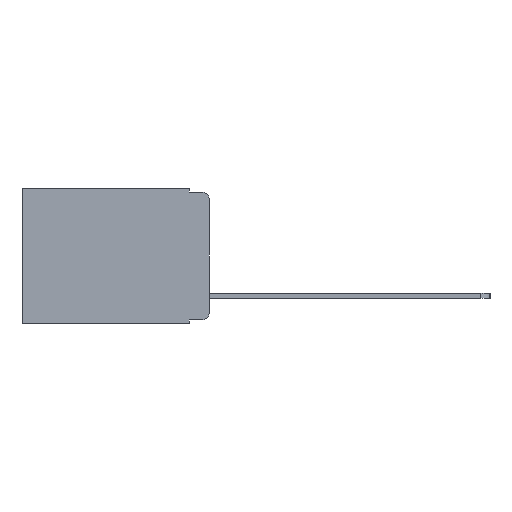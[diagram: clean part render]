
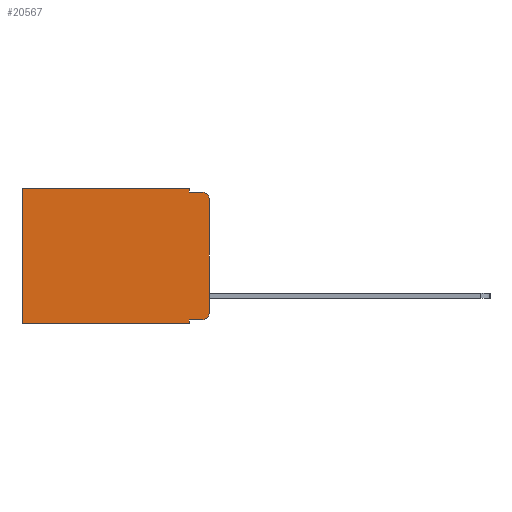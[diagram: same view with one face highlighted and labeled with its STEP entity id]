
A CAD part, left-side view. The second image highlights one B-rep face of the part: STEP entity #20567.
In plain terms, the highlighted planar face has unit normal (-1, 0, 0).
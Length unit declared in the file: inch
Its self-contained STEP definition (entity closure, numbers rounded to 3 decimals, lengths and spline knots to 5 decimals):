
#244 = PLANE ( 'NONE',  #8494 ) ;
#344 = CARTESIAN_POINT ( 'NONE',  ( 0.298, 0.473, 0. ) ) ;
#379 = CARTESIAN_POINT ( 'NONE',  ( 0.298, 0.051, -0.333 ) ) ;
#844 = EDGE_CURVE ( 'NONE', #4341, #19046, #16260, .T. ) ;
#887 = VECTOR ( 'NONE', #14789, 39.37008 ) ;
#1868 = VECTOR ( 'NONE', #18567, 39.37008 ) ;
#2318 = LINE ( 'NONE', #379, #11775 ) ;
#2356 = VERTEX_POINT ( 'NONE', #9933 ) ;
#2668 = DIRECTION ( 'NONE',  ( -1., 0., 0. ) ) ;
#3443 = VECTOR ( 'NONE', #21147, 39.37008 ) ;
#3569 = EDGE_LOOP ( 'NONE', ( #6700, #14458, #13528, #19645, #6907, #20405, #20535, #8109, #5066, #17467 ) ) ;
#4010 = EDGE_CURVE ( 'NONE', #9121, #9765, #20367, .T. ) ;
#4024 = LINE ( 'NONE', #5365, #3443 ) ;
#4341 = VERTEX_POINT ( 'NONE', #8606 ) ;
#4389 = FACE_OUTER_BOUND ( 'NONE', #3569, .T. ) ;
#4958 = CARTESIAN_POINT ( 'NONE',  ( 0.298, 0., 0. ) ) ;
#5066 = ORIENTED_EDGE ( 'NONE', *, *, #10896, .T. ) ;
#5077 = LINE ( 'NONE', #14266, #9252 ) ;
#5365 = CARTESIAN_POINT ( 'NONE',  ( 0.298, 0.473, 0. ) ) ;
#5915 = CARTESIAN_POINT ( 'NONE',  ( 0.298, 0., 0. ) ) ;
#6118 = CARTESIAN_POINT ( 'NONE',  ( 0.298, 0.051, -0.343 ) ) ;
#6130 = VERTEX_POINT ( 'NONE', #8306 ) ;
#6518 = VECTOR ( 'NONE', #14346, 39.37008 ) ;
#6700 = ORIENTED_EDGE ( 'NONE', *, *, #844, .F. ) ;
#6907 = ORIENTED_EDGE ( 'NONE', *, *, #4010, .T. ) ;
#7292 = CARTESIAN_POINT ( 'NONE',  ( 0.298, 0.02, -0.01 ) ) ;
#7557 = CARTESIAN_POINT ( 'NONE',  ( 0.298, 0., 0. ) ) ;
#7899 = DIRECTION ( 'NONE',  ( -1., 0., 0. ) ) ;
#8109 = ORIENTED_EDGE ( 'NONE', *, *, #12081, .F. ) ;
#8306 = CARTESIAN_POINT ( 'NONE',  ( 0.298, 0.051, -0.333 ) ) ;
#8329 = VERTEX_POINT ( 'NONE', #10841 ) ;
#8494 = AXIS2_PLACEMENT_3D ( 'NONE', #7557, #19866, #9335 ) ;
#8558 = EDGE_CURVE ( 'NONE', #8329, #19046, #20690, .T. ) ;
#8606 = CARTESIAN_POINT ( 'NONE',  ( 0.298, 0., -0.03 ) ) ;
#9121 = VERTEX_POINT ( 'NONE', #21879 ) ;
#9252 = VECTOR ( 'NONE', #12483, 39.37008 ) ;
#9256 = VERTEX_POINT ( 'NONE', #6118 ) ;
#9335 = DIRECTION ( 'NONE',  ( 0., 0., -1. ) ) ;
#9765 = VERTEX_POINT ( 'NONE', #344 ) ;
#9933 = CARTESIAN_POINT ( 'NONE',  ( 0.298, 0.473, -0.343 ) ) ;
#10841 = CARTESIAN_POINT ( 'NONE',  ( 0.298, 0.02, -0.333 ) ) ;
#10896 = EDGE_CURVE ( 'NONE', #6130, #8329, #2318, .T. ) ;
#11553 = VECTOR ( 'NONE', #13019, 39.37008 ) ;
#11775 = VECTOR ( 'NONE', #12902, 39.37008 ) ;
#12081 = EDGE_CURVE ( 'NONE', #6130, #9256, #5077, .T. ) ;
#12270 = CARTESIAN_POINT ( 'NONE',  ( 0.298, 0., -0.313 ) ) ;
#12402 = VERTEX_POINT ( 'NONE', #20801 ) ;
#12483 = DIRECTION ( 'NONE',  ( 0., 0., -1. ) ) ;
#12562 = CARTESIAN_POINT ( 'NONE',  ( 0.298, 0.051, 0. ) ) ;
#12902 = DIRECTION ( 'NONE',  ( 0., -1., 0. ) ) ;
#13019 = DIRECTION ( 'NONE',  ( 0., 0., -1. ) ) ;
#13246 = CARTESIAN_POINT ( 'NONE',  ( 0.298, 0.051, -0.01 ) ) ;
#13308 = CARTESIAN_POINT ( 'NONE',  ( 0.298, 0.02, -0.313 ) ) ;
#13528 = ORIENTED_EDGE ( 'NONE', *, *, #19177, .F. ) ;
#14266 = CARTESIAN_POINT ( 'NONE',  ( 0.298, 0.051, 0. ) ) ;
#14346 = DIRECTION ( 'NONE',  ( 0., 0., -1. ) ) ;
#14458 = ORIENTED_EDGE ( 'NONE', *, *, #20362, .T. ) ;
#14789 = DIRECTION ( 'NONE',  ( 0., 1., 0. ) ) ;
#15082 = DIRECTION ( 'NONE',  ( 0., 0., -1. ) ) ;
#15508 = LINE ( 'NONE', #13246, #1868 ) ;
#15643 = EDGE_CURVE ( 'NONE', #9765, #2356, #4024, .T. ) ;
#15865 = CARTESIAN_POINT ( 'NONE',  ( 0.298, 0., -0.343 ) ) ;
#15909 = LINE ( 'NONE', #12562, #6518 ) ;
#15942 = DIRECTION ( 'NONE',  ( 0., 1., 0. ) ) ;
#16016 = AXIS2_PLACEMENT_3D ( 'NONE', #18449, #7899, #20206 ) ;
#16260 = LINE ( 'NONE', #4958, #11553 ) ;
#16822 = EDGE_CURVE ( 'NONE', #9121, #12402, #15909, .T. ) ;
#17467 = ORIENTED_EDGE ( 'NONE', *, *, #8558, .T. ) ;
#18200 = CIRCLE ( 'NONE', #16016, 0.02 ) ;
#18240 = VECTOR ( 'NONE', #15942, 39.37008 ) ;
#18449 = CARTESIAN_POINT ( 'NONE',  ( 0.298, 0.02, -0.03 ) ) ;
#18567 = DIRECTION ( 'NONE',  ( 0., -1., 0. ) ) ;
#19046 = VERTEX_POINT ( 'NONE', #12270 ) ;
#19177 = EDGE_CURVE ( 'NONE', #12402, #20173, #15508, .T. ) ;
#19488 = EDGE_CURVE ( 'NONE', #9256, #2356, #22865, .T. ) ;
#19645 = ORIENTED_EDGE ( 'NONE', *, *, #16822, .F. ) ;
#19838 = AXIS2_PLACEMENT_3D ( 'NONE', #13308, #2668, #15082 ) ;
#19866 = DIRECTION ( 'NONE',  ( 1., 0., 0. ) ) ;
#20173 = VERTEX_POINT ( 'NONE', #7292 ) ;
#20206 = DIRECTION ( 'NONE',  ( 0., 0., -1. ) ) ;
#20362 = EDGE_CURVE ( 'NONE', #4341, #20173, #18200, .T. ) ;
#20367 = LINE ( 'NONE', #5915, #887 ) ;
#20405 = ORIENTED_EDGE ( 'NONE', *, *, #15643, .T. ) ;
#20535 = ORIENTED_EDGE ( 'NONE', *, *, #19488, .F. ) ;
#20567 = ADVANCED_FACE ( 'NONE', ( #4389 ), #244, .F. ) ;
#20690 = CIRCLE ( 'NONE', #19838, 0.02 ) ;
#20801 = CARTESIAN_POINT ( 'NONE',  ( 0.298, 0.051, -0.01 ) ) ;
#21147 = DIRECTION ( 'NONE',  ( 0., 0., -1. ) ) ;
#21879 = CARTESIAN_POINT ( 'NONE',  ( 0.298, 0.051, 0. ) ) ;
#22865 = LINE ( 'NONE', #15865, #18240 ) ;
